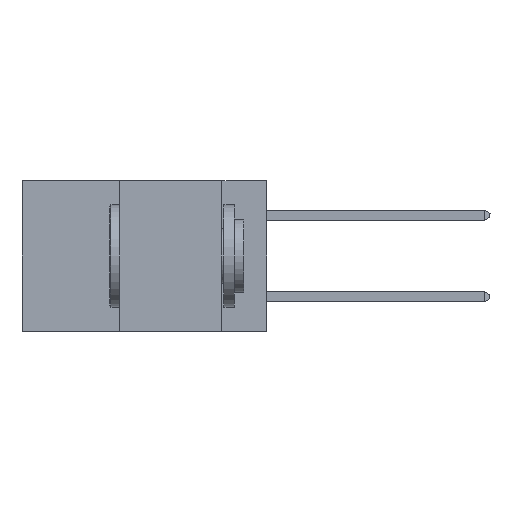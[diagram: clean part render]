
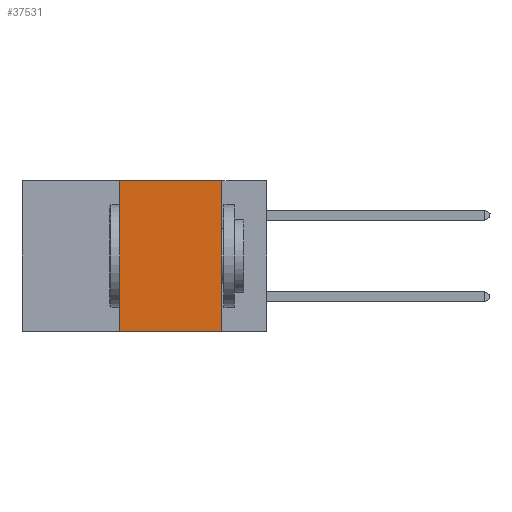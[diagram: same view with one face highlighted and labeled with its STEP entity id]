
A CAD part, left-side view. The second image highlights one B-rep face of the part: STEP entity #37531.
In plain terms, the highlighted planar face has unit normal (-1, 0, 0).
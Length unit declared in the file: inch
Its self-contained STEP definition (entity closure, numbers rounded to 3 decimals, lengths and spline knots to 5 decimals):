
#558 = DIRECTION ( 'NONE',  ( 1., 0., 0. ) ) ;
#1637 = ORIENTED_EDGE ( 'NONE', *, *, #19043, .T. ) ;
#2508 = VECTOR ( 'NONE', #3912, 39.37008 ) ;
#3912 = DIRECTION ( 'NONE',  ( 0., -1., 0. ) ) ;
#5659 = DIRECTION ( 'NONE',  ( 0., 0., 1. ) ) ;
#6950 = LINE ( 'NONE', #20146, #28225 ) ;
#7904 = EDGE_CURVE ( 'NONE', #14136, #37390, #37856, .T. ) ;
#8121 = DIRECTION ( 'NONE',  ( 0., -1., 0. ) ) ;
#8181 = EDGE_CURVE ( 'NONE', #37390, #27834, #34600, .T. ) ;
#9187 = CARTESIAN_POINT ( 'NONE',  ( 0., 0.11, -0.37 ) ) ;
#13113 = DIRECTION ( 'NONE',  ( 0., 0., -1. ) ) ;
#13368 = VECTOR ( 'NONE', #13113, 39.37008 ) ;
#14136 = VERTEX_POINT ( 'NONE', #24097 ) ;
#14346 = CARTESIAN_POINT ( 'NONE',  ( 0., 0.11, 0. ) ) ;
#14834 = ORIENTED_EDGE ( 'NONE', *, *, #8181, .F. ) ;
#14902 = VERTEX_POINT ( 'NONE', #9187 ) ;
#15626 = PLANE ( 'NONE',  #24598 ) ;
#16743 = ORIENTED_EDGE ( 'NONE', *, *, #7904, .F. ) ;
#18955 = CARTESIAN_POINT ( 'NONE',  ( 0., 0.6, 0. ) ) ;
#19043 = EDGE_CURVE ( 'NONE', #14136, #14902, #6950, .T. ) ;
#19215 = CARTESIAN_POINT ( 'NONE',  ( 0., 0.11, 0. ) ) ;
#20146 = CARTESIAN_POINT ( 'NONE',  ( 0., 0.6, -0.37 ) ) ;
#21730 = DIRECTION ( 'NONE',  ( 0., 0., -1. ) ) ;
#22664 = FACE_OUTER_BOUND ( 'NONE', #33831, .T. ) ;
#23639 = CARTESIAN_POINT ( 'NONE',  ( 0., 0.36, 0. ) ) ;
#23653 = EDGE_CURVE ( 'NONE', #27834, #14902, #27601, .T. ) ;
#24097 = CARTESIAN_POINT ( 'NONE',  ( 0., 0.36, -0.37 ) ) ;
#24598 = AXIS2_PLACEMENT_3D ( 'NONE', #36699, #558, #21730 ) ;
#26200 = VECTOR ( 'NONE', #5659, 39.37008 ) ;
#26521 = CARTESIAN_POINT ( 'NONE',  ( 0., 0.36, 0. ) ) ;
#27601 = LINE ( 'NONE', #19215, #13368 ) ;
#27834 = VERTEX_POINT ( 'NONE', #14346 ) ;
#28225 = VECTOR ( 'NONE', #8121, 39.37008 ) ;
#33831 = EDGE_LOOP ( 'NONE', ( #37898, #14834, #16743, #1637 ) ) ;
#34600 = LINE ( 'NONE', #18955, #2508 ) ;
#36699 = CARTESIAN_POINT ( 'NONE',  ( 0., 0.6, 0. ) ) ;
#37390 = VERTEX_POINT ( 'NONE', #26521 ) ;
#37531 = ADVANCED_FACE ( 'NONE', ( #22664 ), #15626, .F. ) ;
#37856 = LINE ( 'NONE', #23639, #26200 ) ;
#37898 = ORIENTED_EDGE ( 'NONE', *, *, #23653, .F. ) ;
